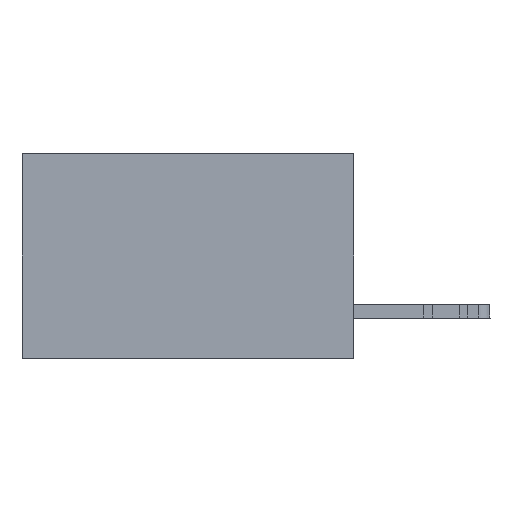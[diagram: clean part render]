
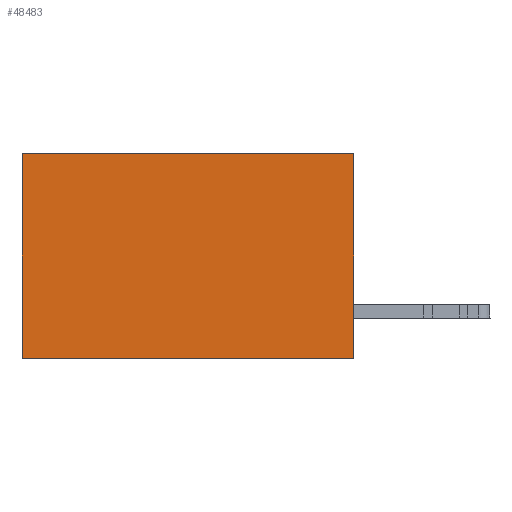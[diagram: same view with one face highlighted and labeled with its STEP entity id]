
A CAD part, left-side view. The second image highlights one B-rep face of the part: STEP entity #48483.
In plain terms, the highlighted planar face has unit normal (-1, 0, 0).
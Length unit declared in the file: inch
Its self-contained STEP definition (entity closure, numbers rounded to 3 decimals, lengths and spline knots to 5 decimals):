
#3411 = DIRECTION ( 'NONE',  ( 0., 0., -1. ) ) ;
#3677 = CARTESIAN_POINT ( 'NONE',  ( 0.2875, 0., -0.37 ) ) ;
#3850 = VECTOR ( 'NONE', #39710, 39.37008 ) ;
#4915 = EDGE_CURVE ( 'NONE', #30525, #34246, #47781, .T. ) ;
#5223 = EDGE_LOOP ( 'NONE', ( #16682, #8344, #22264, #33698 ) ) ;
#8344 = ORIENTED_EDGE ( 'NONE', *, *, #4915, .F. ) ;
#11606 = DIRECTION ( 'NONE',  ( 1., 0., 0. ) ) ;
#15401 = CARTESIAN_POINT ( 'NONE',  ( 0.2875, 0., 0. ) ) ;
#15961 = VECTOR ( 'NONE', #36295, 39.37008 ) ;
#16682 = ORIENTED_EDGE ( 'NONE', *, *, #28894, .T. ) ;
#17373 = VECTOR ( 'NONE', #19269, 39.37008 ) ;
#19269 = DIRECTION ( 'NONE',  ( 0., 1., 0. ) ) ;
#20041 = FACE_OUTER_BOUND ( 'NONE', #5223, .T. ) ;
#22264 = ORIENTED_EDGE ( 'NONE', *, *, #32077, .F. ) ;
#23170 = CARTESIAN_POINT ( 'NONE',  ( 0.2875, 0., 0. ) ) ;
#23939 = VECTOR ( 'NONE', #45049, 39.37008 ) ;
#25875 = CARTESIAN_POINT ( 'NONE',  ( 0.2875, 0., 0. ) ) ;
#26240 = CARTESIAN_POINT ( 'NONE',  ( 0.2875, 0.6, -0.37 ) ) ;
#26535 = PLANE ( 'NONE',  #31247 ) ;
#28894 = EDGE_CURVE ( 'NONE', #43490, #34246, #42888, .T. ) ;
#29072 = CARTESIAN_POINT ( 'NONE',  ( 0.2875, 0., 0. ) ) ;
#30410 = VERTEX_POINT ( 'NONE', #23170 ) ;
#30525 = VERTEX_POINT ( 'NONE', #39858 ) ;
#31247 = AXIS2_PLACEMENT_3D ( 'NONE', #25875, #11606, #3411 ) ;
#31275 = EDGE_CURVE ( 'NONE', #30410, #43490, #37398, .T. ) ;
#32061 = LINE ( 'NONE', #29072, #3850 ) ;
#32077 = EDGE_CURVE ( 'NONE', #30410, #30525, #32061, .T. ) ;
#33698 = ORIENTED_EDGE ( 'NONE', *, *, #31275, .T. ) ;
#34246 = VERTEX_POINT ( 'NONE', #26240 ) ;
#34956 = CARTESIAN_POINT ( 'NONE',  ( 0.2875, 0.6, 0. ) ) ;
#36295 = DIRECTION ( 'NONE',  ( 0., 0., -1. ) ) ;
#37398 = LINE ( 'NONE', #15401, #23939 ) ;
#39710 = DIRECTION ( 'NONE',  ( 0., 0., -1. ) ) ;
#39858 = CARTESIAN_POINT ( 'NONE',  ( 0.2875, 0., -0.37 ) ) ;
#40397 = CARTESIAN_POINT ( 'NONE',  ( 0.2875, 0.6, 0. ) ) ;
#42888 = LINE ( 'NONE', #40397, #15961 ) ;
#43490 = VERTEX_POINT ( 'NONE', #34956 ) ;
#45049 = DIRECTION ( 'NONE',  ( 0., 1., 0. ) ) ;
#47781 = LINE ( 'NONE', #3677, #17373 ) ;
#48483 = ADVANCED_FACE ( 'NONE', ( #20041 ), #26535, .F. ) ;
